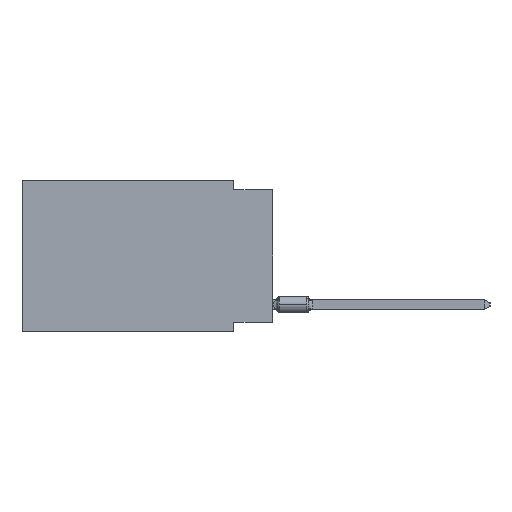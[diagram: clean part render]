
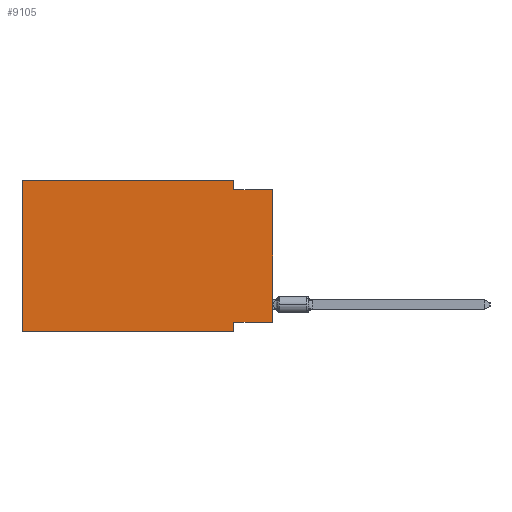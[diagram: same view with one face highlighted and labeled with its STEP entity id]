
A CAD part, left-side view. The second image highlights one B-rep face of the part: STEP entity #9105.
In plain terms, the highlighted planar face has unit normal (-1, 0, 0).
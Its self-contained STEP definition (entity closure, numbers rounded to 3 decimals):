
#571 = VERTEX_POINT ( 'NONE', #45534 ) ;
#699 = CARTESIAN_POINT ( 'NONE',  ( 0., 16.383, 0. ) ) ;
#812 = VECTOR ( 'NONE', #1694, 1000. ) ;
#1694 = DIRECTION ( 'NONE',  ( 0., -1., 0. ) ) ;
#1876 = EDGE_CURVE ( 'NONE', #28787, #56231, #53031, .T. ) ;
#2332 = VECTOR ( 'NONE', #9253, 1000. ) ;
#3561 = CARTESIAN_POINT ( 'NONE',  ( 0., 16.383, -9.906 ) ) ;
#3651 = VERTEX_POINT ( 'NONE', #28809 ) ;
#4155 = DIRECTION ( 'NONE',  ( 0., 0., -1. ) ) ;
#4871 = CARTESIAN_POINT ( 'NONE',  ( 0., 2.54, -9.906 ) ) ;
#5713 = LINE ( 'NONE', #4871, #22928 ) ;
#5925 = DIRECTION ( 'NONE',  ( 0., 0., 1. ) ) ;
#7638 = CARTESIAN_POINT ( 'NONE',  ( 0., 16.383, 0. ) ) ;
#7927 = ORIENTED_EDGE ( 'NONE', *, *, #54595, .F. ) ;
#8347 = VERTEX_POINT ( 'NONE', #54331 ) ;
#9105 = ADVANCED_FACE ( 'NONE', ( #43374 ), #39376, .F. ) ;
#9253 = DIRECTION ( 'NONE',  ( 0., -1., 0. ) ) ;
#9584 = CARTESIAN_POINT ( 'NONE',  ( 0., 0., -9.271 ) ) ;
#11682 = DIRECTION ( 'NONE',  ( 0., 0., -1. ) ) ;
#12308 = AXIS2_PLACEMENT_3D ( 'NONE', #699, #43944, #4155 ) ;
#16567 = EDGE_CURVE ( 'NONE', #31510, #8347, #45542, .T. ) ;
#16850 = ORIENTED_EDGE ( 'NONE', *, *, #27469, .F. ) ;
#17113 = CARTESIAN_POINT ( 'NONE',  ( 0., 2.54, 0. ) ) ;
#17588 = CARTESIAN_POINT ( 'NONE',  ( 0., 2.54, -9.906 ) ) ;
#19760 = DIRECTION ( 'NONE',  ( 0., -1., 0. ) ) ;
#21376 = DIRECTION ( 'NONE',  ( 0., 0., 1. ) ) ;
#22928 = VECTOR ( 'NONE', #23185, 1000. ) ;
#23185 = DIRECTION ( 'NONE',  ( 0., 0., -1. ) ) ;
#24662 = EDGE_CURVE ( 'NONE', #42178, #3651, #28521, .T. ) ;
#25275 = EDGE_CURVE ( 'NONE', #571, #3651, #43915, .T. ) ;
#27469 = EDGE_CURVE ( 'NONE', #50564, #56231, #5713, .T. ) ;
#28521 = LINE ( 'NONE', #45435, #50769 ) ;
#28787 = VERTEX_POINT ( 'NONE', #3561 ) ;
#28809 = CARTESIAN_POINT ( 'NONE',  ( 0., 0., -0.635 ) ) ;
#31510 = VERTEX_POINT ( 'NONE', #51721 ) ;
#32516 = VECTOR ( 'NONE', #21376, 1000. ) ;
#33890 = ORIENTED_EDGE ( 'NONE', *, *, #1876, .T. ) ;
#36949 = CARTESIAN_POINT ( 'NONE',  ( 0., 16.383, 0. ) ) ;
#38281 = ORIENTED_EDGE ( 'NONE', *, *, #43031, .F. ) ;
#39376 = PLANE ( 'NONE',  #12308 ) ;
#41523 = VECTOR ( 'NONE', #11682, 1000. ) ;
#42178 = VERTEX_POINT ( 'NONE', #43302 ) ;
#43031 = EDGE_CURVE ( 'NONE', #8347, #571, #56344, .T. ) ;
#43302 = CARTESIAN_POINT ( 'NONE',  ( 0., 0., -9.271 ) ) ;
#43374 = FACE_OUTER_BOUND ( 'NONE', #48103, .T. ) ;
#43915 = LINE ( 'NONE', #48489, #2332 ) ;
#43944 = DIRECTION ( 'NONE',  ( 1., 0., 0. ) ) ;
#44521 = LINE ( 'NONE', #9584, #45006 ) ;
#45006 = VECTOR ( 'NONE', #48541, 1000. ) ;
#45435 = CARTESIAN_POINT ( 'NONE',  ( 0., 0., 0. ) ) ;
#45477 = EDGE_CURVE ( 'NONE', #42178, #50564, #44521, .T. ) ;
#45534 = CARTESIAN_POINT ( 'NONE',  ( 0., 2.54, -0.635 ) ) ;
#45542 = LINE ( 'NONE', #36949, #49250 ) ;
#45612 = CARTESIAN_POINT ( 'NONE',  ( 0., 2.54, -9.271 ) ) ;
#46861 = LINE ( 'NONE', #7638, #32516 ) ;
#48103 = EDGE_LOOP ( 'NONE', ( #54383, #51872, #38281, #54337, #7927, #33890, #16850, #53984 ) ) ;
#48489 = CARTESIAN_POINT ( 'NONE',  ( 0., 0., -0.635 ) ) ;
#48541 = DIRECTION ( 'NONE',  ( 0., 1., 0. ) ) ;
#48731 = CARTESIAN_POINT ( 'NONE',  ( 0., 16.383, -9.906 ) ) ;
#49250 = VECTOR ( 'NONE', #19760, 1000. ) ;
#50564 = VERTEX_POINT ( 'NONE', #45612 ) ;
#50769 = VECTOR ( 'NONE', #5925, 1000. ) ;
#51721 = CARTESIAN_POINT ( 'NONE',  ( 0., 16.383, 0. ) ) ;
#51872 = ORIENTED_EDGE ( 'NONE', *, *, #25275, .F. ) ;
#53031 = LINE ( 'NONE', #48731, #812 ) ;
#53984 = ORIENTED_EDGE ( 'NONE', *, *, #45477, .F. ) ;
#54331 = CARTESIAN_POINT ( 'NONE',  ( 0., 2.54, 0. ) ) ;
#54337 = ORIENTED_EDGE ( 'NONE', *, *, #16567, .F. ) ;
#54383 = ORIENTED_EDGE ( 'NONE', *, *, #24662, .T. ) ;
#54595 = EDGE_CURVE ( 'NONE', #28787, #31510, #46861, .T. ) ;
#56231 = VERTEX_POINT ( 'NONE', #17588 ) ;
#56344 = LINE ( 'NONE', #17113, #41523 ) ;
